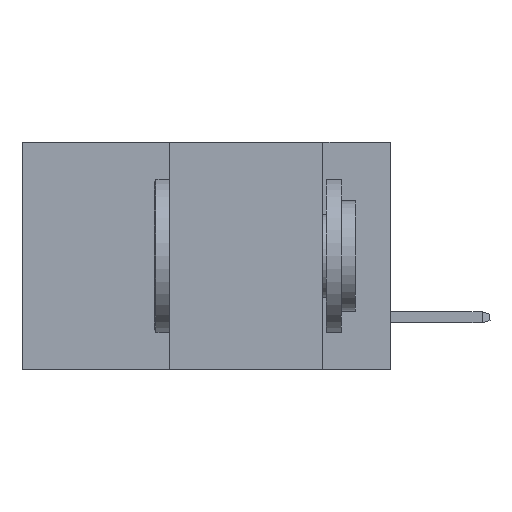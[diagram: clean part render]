
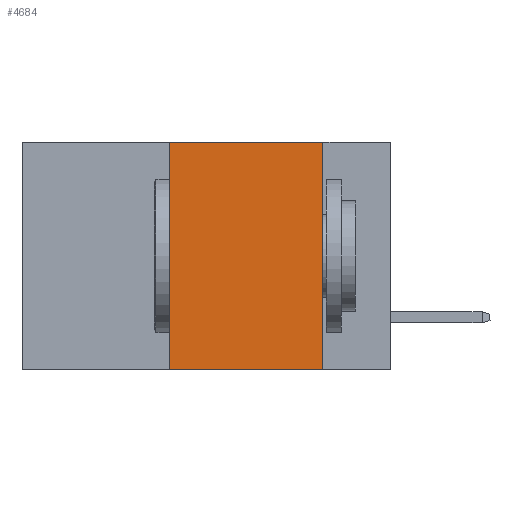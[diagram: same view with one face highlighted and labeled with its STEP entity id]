
A CAD part, left-side view. The second image highlights one B-rep face of the part: STEP entity #4684.
In plain terms, the highlighted planar face has unit normal (-1, 0, 0).
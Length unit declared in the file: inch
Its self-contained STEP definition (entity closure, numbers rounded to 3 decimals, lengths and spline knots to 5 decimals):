
#101 = CARTESIAN_POINT ( 'NONE',  ( 0., 0.6, 0. ) ) ;
#577 = VERTEX_POINT ( 'NONE', #10074 ) ;
#879 = AXIS2_PLACEMENT_3D ( 'NONE', #101, #13614, #13502 ) ;
#883 = VERTEX_POINT ( 'NONE', #15667 ) ;
#1371 = VECTOR ( 'NONE', #14244, 39.37008 ) ;
#2906 = ORIENTED_EDGE ( 'NONE', *, *, #8502, .F. ) ;
#4087 = VERTEX_POINT ( 'NONE', #15466 ) ;
#4398 = EDGE_CURVE ( 'NONE', #883, #4087, #4907, .T. ) ;
#4472 = CARTESIAN_POINT ( 'NONE',  ( 0., 0.6, 0. ) ) ;
#4684 = ADVANCED_FACE ( 'NONE', ( #4930 ), #17904, .F. ) ;
#4907 = LINE ( 'NONE', #14305, #1371 ) ;
#4930 = FACE_OUTER_BOUND ( 'NONE', #8733, .T. ) ;
#5948 = DIRECTION ( 'NONE',  ( 0., -1., 0. ) ) ;
#6147 = VECTOR ( 'NONE', #5948, 39.37008 ) ;
#7185 = CARTESIAN_POINT ( 'NONE',  ( 0., 0.36, 0. ) ) ;
#7266 = VECTOR ( 'NONE', #8738, 39.37008 ) ;
#8237 = ORIENTED_EDGE ( 'NONE', *, *, #4398, .T. ) ;
#8502 = EDGE_CURVE ( 'NONE', #13712, #577, #10283, .T. ) ;
#8733 = EDGE_LOOP ( 'NONE', ( #11927, #2906, #12149, #8237 ) ) ;
#8738 = DIRECTION ( 'NONE',  ( 0., 0., 1. ) ) ;
#9418 = CARTESIAN_POINT ( 'NONE',  ( 0., 0.11, 0. ) ) ;
#9422 = EDGE_CURVE ( 'NONE', #577, #4087, #13044, .T. ) ;
#10074 = CARTESIAN_POINT ( 'NONE',  ( 0., 0.11, 0. ) ) ;
#10283 = LINE ( 'NONE', #4472, #6147 ) ;
#10966 = LINE ( 'NONE', #18197, #7266 ) ;
#11927 = ORIENTED_EDGE ( 'NONE', *, *, #9422, .F. ) ;
#12149 = ORIENTED_EDGE ( 'NONE', *, *, #15024, .F. ) ;
#12185 = DIRECTION ( 'NONE',  ( 0., 0., -1. ) ) ;
#12619 = VECTOR ( 'NONE', #12185, 39.37008 ) ;
#13044 = LINE ( 'NONE', #9418, #12619 ) ;
#13502 = DIRECTION ( 'NONE',  ( 0., 0., -1. ) ) ;
#13614 = DIRECTION ( 'NONE',  ( 1., 0., 0. ) ) ;
#13712 = VERTEX_POINT ( 'NONE', #7185 ) ;
#14244 = DIRECTION ( 'NONE',  ( 0., -1., 0. ) ) ;
#14305 = CARTESIAN_POINT ( 'NONE',  ( 0., 0.6, -0.37 ) ) ;
#15024 = EDGE_CURVE ( 'NONE', #883, #13712, #10966, .T. ) ;
#15466 = CARTESIAN_POINT ( 'NONE',  ( 0., 0.11, -0.37 ) ) ;
#15667 = CARTESIAN_POINT ( 'NONE',  ( 0., 0.36, -0.37 ) ) ;
#17904 = PLANE ( 'NONE',  #879 ) ;
#18197 = CARTESIAN_POINT ( 'NONE',  ( 0., 0.36, 0. ) ) ;
